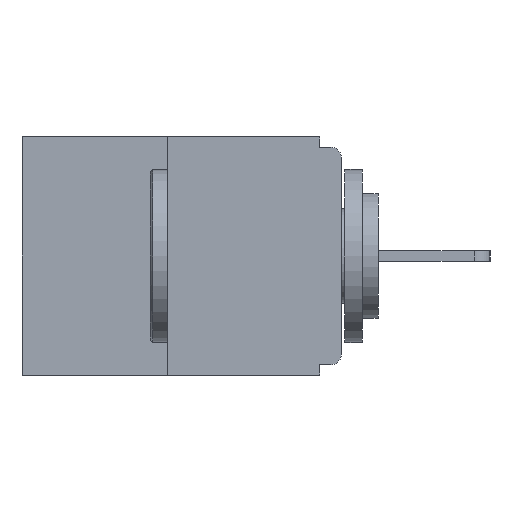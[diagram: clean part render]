
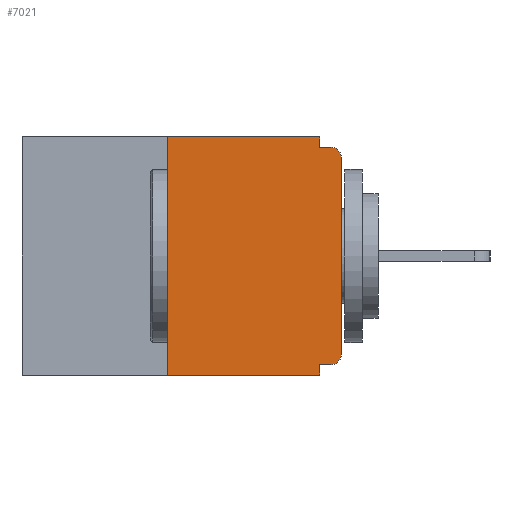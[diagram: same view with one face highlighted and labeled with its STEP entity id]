
A CAD part, left-side view. The second image highlights one B-rep face of the part: STEP entity #7021.
In plain terms, the highlighted planar face has unit normal (-1, 0, 0).
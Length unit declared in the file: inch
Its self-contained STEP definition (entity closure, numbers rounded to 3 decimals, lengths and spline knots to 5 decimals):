
#21 = VERTEX_POINT ( 'NONE', #16946 ) ;
#56 = ORIENTED_EDGE ( 'NONE', *, *, #26250, .T. ) ;
#451 = DIRECTION ( 'NONE',  ( -1., 0., 0. ) ) ;
#509 = PLANE ( 'NONE',  #21402 ) ;
#703 = DIRECTION ( 'NONE',  ( 0., 0., 1. ) ) ;
#727 = EDGE_CURVE ( 'NONE', #916, #10930, #3923, .T. ) ;
#861 = EDGE_CURVE ( 'NONE', #22280, #26084, #21856, .T. ) ;
#916 = VERTEX_POINT ( 'NONE', #19844 ) ;
#1213 = ORIENTED_EDGE ( 'NONE', *, *, #27140, .T. ) ;
#1235 = DIRECTION ( 'NONE',  ( -1., 0., 0. ) ) ;
#1546 = CARTESIAN_POINT ( 'NONE',  ( 0., 0.031, -0.343 ) ) ;
#1634 = ORIENTED_EDGE ( 'NONE', *, *, #7866, .F. ) ;
#2480 = CARTESIAN_POINT ( 'NONE',  ( 0., 0.015, -0.03 ) ) ;
#2799 = LINE ( 'NONE', #9081, #3212 ) ;
#2817 = ORIENTED_EDGE ( 'NONE', *, *, #4132, .F. ) ;
#3103 = DIRECTION ( 'NONE',  ( 0., 0., -1. ) ) ;
#3212 = VECTOR ( 'NONE', #22373, 39.37008 ) ;
#3923 = LINE ( 'NONE', #22913, #13443 ) ;
#4132 = EDGE_CURVE ( 'NONE', #8830, #21761, #12545, .T. ) ;
#5927 = CIRCLE ( 'NONE', #7711, 0.015 ) ;
#7021 = ADVANCED_FACE ( 'NONE', ( #15544 ), #509, .F. ) ;
#7711 = AXIS2_PLACEMENT_3D ( 'NONE', #10900, #451, #17291 ) ;
#7866 = EDGE_CURVE ( 'NONE', #24644, #916, #18084, .T. ) ;
#8256 = DIRECTION ( 'NONE',  ( 0., 0., -1. ) ) ;
#8283 = VERTEX_POINT ( 'NONE', #11483 ) ;
#8480 = LINE ( 'NONE', #14546, #17641 ) ;
#8830 = VERTEX_POINT ( 'NONE', #16841 ) ;
#9081 = CARTESIAN_POINT ( 'NONE',  ( 0., 0., 0. ) ) ;
#9279 = CARTESIAN_POINT ( 'NONE',  ( 0., 0.25, 0. ) ) ;
#9530 = LINE ( 'NONE', #19846, #24457 ) ;
#9602 = EDGE_CURVE ( 'NONE', #20195, #8830, #8480, .T. ) ;
#9699 = EDGE_CURVE ( 'NONE', #10930, #21, #15067, .T. ) ;
#9739 = CARTESIAN_POINT ( 'NONE',  ( 0., 0.46, -0.343 ) ) ;
#10209 = CARTESIAN_POINT ( 'NONE',  ( 0., 0.031, 0. ) ) ;
#10251 = VECTOR ( 'NONE', #27149, 39.37008 ) ;
#10338 = CARTESIAN_POINT ( 'NONE',  ( 0., 0.031, -0.343 ) ) ;
#10867 = DIRECTION ( 'NONE',  ( 0., 0., -1. ) ) ;
#10900 = CARTESIAN_POINT ( 'NONE',  ( 0., 0.015, -0.313 ) ) ;
#10930 = VERTEX_POINT ( 'NONE', #10209 ) ;
#11208 = CARTESIAN_POINT ( 'NONE',  ( 0., 0.46, 0. ) ) ;
#11350 = DIRECTION ( 'NONE',  ( 1., 0., 0. ) ) ;
#11483 = CARTESIAN_POINT ( 'NONE',  ( 0., 0., -0.313 ) ) ;
#11670 = ORIENTED_EDGE ( 'NONE', *, *, #9699, .F. ) ;
#11975 = LINE ( 'NONE', #9739, #10251 ) ;
#12394 = ORIENTED_EDGE ( 'NONE', *, *, #9602, .F. ) ;
#12401 = DIRECTION ( 'NONE',  ( 0., -1., 0. ) ) ;
#12545 = LINE ( 'NONE', #10338, #18642 ) ;
#12853 = EDGE_CURVE ( 'NONE', #21, #26084, #9530, .T. ) ;
#13443 = VECTOR ( 'NONE', #12401, 39.37008 ) ;
#13689 = CARTESIAN_POINT ( 'NONE',  ( 0., 0.015, -0.328 ) ) ;
#13781 = DIRECTION ( 'NONE',  ( 0., -1., 0. ) ) ;
#14071 = CARTESIAN_POINT ( 'NONE',  ( 0., 0.015, -0.015 ) ) ;
#14546 = CARTESIAN_POINT ( 'NONE',  ( 0., 0., -0.328 ) ) ;
#14768 = AXIS2_PLACEMENT_3D ( 'NONE', #2480, #1235, #22431 ) ;
#15067 = LINE ( 'NONE', #21595, #25651 ) ;
#15544 = FACE_OUTER_BOUND ( 'NONE', #21540, .T. ) ;
#16468 = DIRECTION ( 'NONE',  ( 0., 1., 0. ) ) ;
#16841 = CARTESIAN_POINT ( 'NONE',  ( 0., 0.031, -0.328 ) ) ;
#16946 = CARTESIAN_POINT ( 'NONE',  ( 0., 0.031, -0.015 ) ) ;
#17291 = DIRECTION ( 'NONE',  ( 0., 0., -1. ) ) ;
#17641 = VECTOR ( 'NONE', #16468, 39.37008 ) ;
#18084 = LINE ( 'NONE', #9279, #21888 ) ;
#18192 = ORIENTED_EDGE ( 'NONE', *, *, #861, .T. ) ;
#18642 = VECTOR ( 'NONE', #8256, 39.37008 ) ;
#19844 = CARTESIAN_POINT ( 'NONE',  ( 0., 0.25, 0. ) ) ;
#19846 = CARTESIAN_POINT ( 'NONE',  ( 0., 0., -0.015 ) ) ;
#20195 = VERTEX_POINT ( 'NONE', #13689 ) ;
#21330 = EDGE_CURVE ( 'NONE', #24644, #21761, #11975, .T. ) ;
#21402 = AXIS2_PLACEMENT_3D ( 'NONE', #11208, #11350, #3103 ) ;
#21540 = EDGE_LOOP ( 'NONE', ( #22996, #1634, #21899, #2817, #12394, #1213, #56, #18192, #25644, #11670 ) ) ;
#21595 = CARTESIAN_POINT ( 'NONE',  ( 0., 0.031, 0. ) ) ;
#21761 = VERTEX_POINT ( 'NONE', #1546 ) ;
#21856 = CIRCLE ( 'NONE', #14768, 0.015 ) ;
#21888 = VECTOR ( 'NONE', #703, 39.37008 ) ;
#21899 = ORIENTED_EDGE ( 'NONE', *, *, #21330, .T. ) ;
#22280 = VERTEX_POINT ( 'NONE', #25521 ) ;
#22373 = DIRECTION ( 'NONE',  ( 0., 0., 1. ) ) ;
#22431 = DIRECTION ( 'NONE',  ( 0., 0., -1. ) ) ;
#22913 = CARTESIAN_POINT ( 'NONE',  ( 0., 0.46, 0. ) ) ;
#22996 = ORIENTED_EDGE ( 'NONE', *, *, #727, .F. ) ;
#24457 = VECTOR ( 'NONE', #13781, 39.37008 ) ;
#24644 = VERTEX_POINT ( 'NONE', #27058 ) ;
#25521 = CARTESIAN_POINT ( 'NONE',  ( 0., 0., -0.03 ) ) ;
#25644 = ORIENTED_EDGE ( 'NONE', *, *, #12853, .F. ) ;
#25651 = VECTOR ( 'NONE', #10867, 39.37008 ) ;
#26084 = VERTEX_POINT ( 'NONE', #14071 ) ;
#26250 = EDGE_CURVE ( 'NONE', #8283, #22280, #2799, .T. ) ;
#27058 = CARTESIAN_POINT ( 'NONE',  ( 0., 0.25, -0.343 ) ) ;
#27140 = EDGE_CURVE ( 'NONE', #20195, #8283, #5927, .T. ) ;
#27149 = DIRECTION ( 'NONE',  ( 0., -1., 0. ) ) ;
